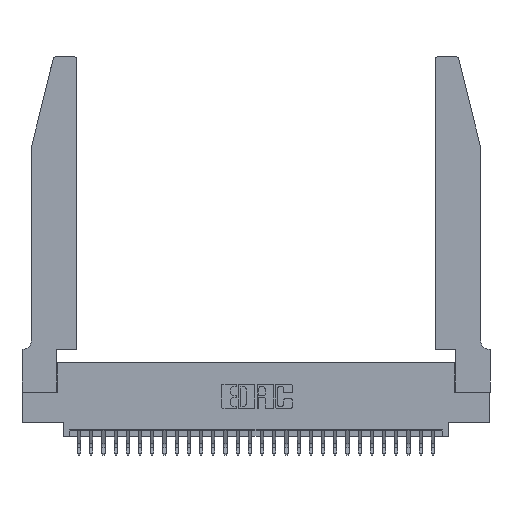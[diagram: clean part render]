
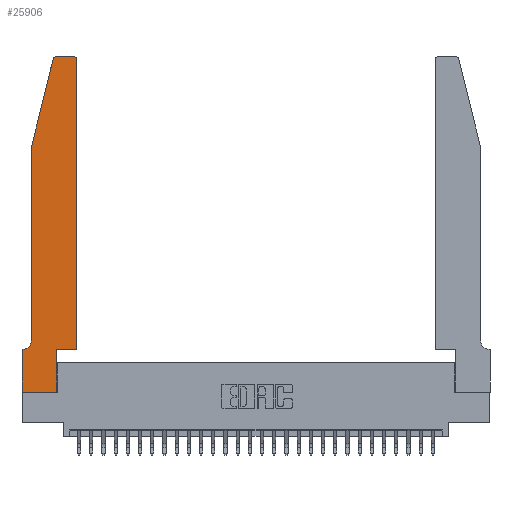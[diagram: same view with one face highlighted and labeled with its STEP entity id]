
A CAD part, top view. The second image highlights one B-rep face of the part: STEP entity #25906.
In plain terms, the highlighted planar face has unit normal (0, 0, 1).
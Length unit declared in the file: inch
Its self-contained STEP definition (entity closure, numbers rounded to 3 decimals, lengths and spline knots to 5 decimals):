
#276 = VECTOR ( 'NONE', #436, 39.37008 ) ;
#436 = DIRECTION ( 'NONE',  ( -1., 0., 0. ) ) ;
#448 = DIRECTION ( 'NONE',  ( 0., 0., 1. ) ) ;
#488 = EDGE_CURVE ( 'NONE', #23680, #1895, #4856, .T. ) ;
#511 = DIRECTION ( 'NONE',  ( 0., 0., 1. ) ) ;
#512 = DIRECTION ( 'NONE',  ( 1., 0., 0. ) ) ;
#603 = EDGE_CURVE ( 'NONE', #10189, #12084, #26690, .T. ) ;
#1034 = PLANE ( 'NONE',  #3310 ) ;
#1354 = DIRECTION ( 'NONE',  ( 0., 0., -1. ) ) ;
#1372 = CARTESIAN_POINT ( 'NONE',  ( 0.4505, 2.72, 0.37 ) ) ;
#1653 = LINE ( 'NONE', #19392, #18982 ) ;
#1687 = CARTESIAN_POINT ( 'NONE',  ( 0.284, 2.72, 0.37 ) ) ;
#1745 = EDGE_CURVE ( 'NONE', #4046, #21541, #2891, .T. ) ;
#1805 = VECTOR ( 'NONE', #23815, 39.37008 ) ;
#1895 = VERTEX_POINT ( 'NONE', #25128 ) ;
#2157 = VECTOR ( 'NONE', #3407, 39.37008 ) ;
#2166 = ORIENTED_EDGE ( 'NONE', *, *, #25799, .T. ) ;
#2244 = ORIENTED_EDGE ( 'NONE', *, *, #603, .T. ) ;
#2560 = EDGE_CURVE ( 'NONE', #2932, #22158, #19732, .T. ) ;
#2891 = LINE ( 'NONE', #7577, #8505 ) ;
#2932 = VERTEX_POINT ( 'NONE', #23604 ) ;
#3072 = EDGE_CURVE ( 'NONE', #22158, #4046, #1653, .T. ) ;
#3310 = AXIS2_PLACEMENT_3D ( 'NONE', #28834, #17592, #3482 ) ;
#3407 = DIRECTION ( 'NONE',  ( -1., 0., 0. ) ) ;
#3482 = DIRECTION ( 'NONE',  ( 1., 0., 0. ) ) ;
#3757 = CARTESIAN_POINT ( 'NONE',  ( 0.4205, 2.75, 0.37 ) ) ;
#4046 = VERTEX_POINT ( 'NONE', #18332 ) ;
#4339 = ORIENTED_EDGE ( 'NONE', *, *, #15029, .T. ) ;
#4535 = VERTEX_POINT ( 'NONE', #1372 ) ;
#4721 = CARTESIAN_POINT ( 'NONE',  ( 0., 0., 0.37 ) ) ;
#4856 = LINE ( 'NONE', #27720, #28850 ) ;
#5128 = ORIENTED_EDGE ( 'NONE', *, *, #22657, .T. ) ;
#5544 = CARTESIAN_POINT ( 'NONE',  ( 0.2865, 0.35, 0.37 ) ) ;
#5922 = CARTESIAN_POINT ( 'NONE',  ( 0.2605, 2.75, 0.37 ) ) ;
#6476 = CARTESIAN_POINT ( 'NONE',  ( 0.4505, 0.35, 0.37 ) ) ;
#7117 = AXIS2_PLACEMENT_3D ( 'NONE', #14786, #511, #17093 ) ;
#7577 = CARTESIAN_POINT ( 'NONE',  ( 0.0755, 2., 0.37 ) ) ;
#8505 = VECTOR ( 'NONE', #15034, 39.37008 ) ;
#8634 = VERTEX_POINT ( 'NONE', #3757 ) ;
#9232 = VECTOR ( 'NONE', #27565, 39.37008 ) ;
#9397 = CARTESIAN_POINT ( 'NONE',  ( 0.4505, 0.35, 0.37 ) ) ;
#10058 = LINE ( 'NONE', #5922, #2157 ) ;
#10189 = VERTEX_POINT ( 'NONE', #13034 ) ;
#10328 = CIRCLE ( 'NONE', #13252, 0.07 ) ;
#11136 = ORIENTED_EDGE ( 'NONE', *, *, #2560, .T. ) ;
#12084 = VERTEX_POINT ( 'NONE', #6476 ) ;
#12278 = VECTOR ( 'NONE', #24158, 39.37008 ) ;
#13034 = CARTESIAN_POINT ( 'NONE',  ( 0.2865, 0.35, 0.37 ) ) ;
#13252 = AXIS2_PLACEMENT_3D ( 'NONE', #15545, #1354, #17889 ) ;
#13412 = ORIENTED_EDGE ( 'NONE', *, *, #3072, .T. ) ;
#13718 = LINE ( 'NONE', #23833, #276 ) ;
#13802 = CARTESIAN_POINT ( 'NONE',  ( 0.4505, 0.35, 0.37 ) ) ;
#14420 = EDGE_CURVE ( 'NONE', #1895, #10189, #29874, .T. ) ;
#14786 = CARTESIAN_POINT ( 'NONE',  ( 0.4205, 2.72, 0.37 ) ) ;
#15029 = EDGE_CURVE ( 'NONE', #12084, #4535, #27680, .T. ) ;
#15034 = DIRECTION ( 'NONE',  ( 0., -1., 0. ) ) ;
#15545 = CARTESIAN_POINT ( 'NONE',  ( 0.0055, 0.42, 0.37 ) ) ;
#16138 = ORIENTED_EDGE ( 'NONE', *, *, #24060, .T. ) ;
#16481 = EDGE_CURVE ( 'NONE', #21570, #23680, #18293, .T. ) ;
#16972 = VERTEX_POINT ( 'NONE', #23539 ) ;
#17092 = DIRECTION ( 'NONE',  ( -0.239, -0.971, 0. ) ) ;
#17093 = DIRECTION ( 'NONE',  ( 1., 0., 0. ) ) ;
#17592 = DIRECTION ( 'NONE',  ( 0., 0., 1. ) ) ;
#17889 = DIRECTION ( 'NONE',  ( -1., 0., 0. ) ) ;
#18293 = LINE ( 'NONE', #4721, #19008 ) ;
#18332 = CARTESIAN_POINT ( 'NONE',  ( 0.0755, 2., 0.37 ) ) ;
#18870 = ORIENTED_EDGE ( 'NONE', *, *, #22479, .T. ) ;
#18982 = VECTOR ( 'NONE', #17092, 39.37008 ) ;
#19008 = VECTOR ( 'NONE', #27893, 39.37008 ) ;
#19392 = CARTESIAN_POINT ( 'NONE',  ( 0.0755, 2., 0.37 ) ) ;
#19732 = CIRCLE ( 'NONE', #29746, 0.03 ) ;
#20115 = DIRECTION ( 'NONE',  ( 1., 0., 0. ) ) ;
#20415 = CIRCLE ( 'NONE', #7117, 0.03 ) ;
#20974 = CARTESIAN_POINT ( 'NONE',  ( 0., 0., 0.37 ) ) ;
#21309 = ORIENTED_EDGE ( 'NONE', *, *, #14420, .T. ) ;
#21541 = VERTEX_POINT ( 'NONE', #22276 ) ;
#21570 = VERTEX_POINT ( 'NONE', #26904 ) ;
#21665 = ORIENTED_EDGE ( 'NONE', *, *, #488, .T. ) ;
#22158 = VERTEX_POINT ( 'NONE', #27063 ) ;
#22276 = CARTESIAN_POINT ( 'NONE',  ( 0.0755, 0.42, 0.37 ) ) ;
#22479 = EDGE_CURVE ( 'NONE', #16972, #21570, #13718, .T. ) ;
#22657 = EDGE_CURVE ( 'NONE', #8634, #2932, #10058, .T. ) ;
#23487 = ORIENTED_EDGE ( 'NONE', *, *, #1745, .T. ) ;
#23539 = CARTESIAN_POINT ( 'NONE',  ( 0.0055, 0.35, 0.37 ) ) ;
#23604 = CARTESIAN_POINT ( 'NONE',  ( 0.284, 2.75, 0.37 ) ) ;
#23680 = VERTEX_POINT ( 'NONE', #20974 ) ;
#23815 = DIRECTION ( 'NONE',  ( 1., 0., 0. ) ) ;
#23833 = CARTESIAN_POINT ( 'NONE',  ( 0.0755, 0.35, 0.37 ) ) ;
#24060 = EDGE_CURVE ( 'NONE', #21541, #16972, #10328, .T. ) ;
#24158 = DIRECTION ( 'NONE',  ( 0., 1., 0. ) ) ;
#25105 = FACE_OUTER_BOUND ( 'NONE', #29223, .T. ) ;
#25128 = CARTESIAN_POINT ( 'NONE',  ( 0.2865, 0., 0.37 ) ) ;
#25799 = EDGE_CURVE ( 'NONE', #4535, #8634, #20415, .T. ) ;
#25906 = ADVANCED_FACE ( 'NONE', ( #25105 ), #1034, .T. ) ;
#26690 = LINE ( 'NONE', #9397, #1805 ) ;
#26904 = CARTESIAN_POINT ( 'NONE',  ( 0., 0.35, 0.37 ) ) ;
#27063 = CARTESIAN_POINT ( 'NONE',  ( 0.25487, 2.72718, 0.37 ) ) ;
#27565 = DIRECTION ( 'NONE',  ( 0., 1., 0. ) ) ;
#27680 = LINE ( 'NONE', #13802, #9232 ) ;
#27720 = CARTESIAN_POINT ( 'NONE',  ( 0., 0., 0.37 ) ) ;
#27893 = DIRECTION ( 'NONE',  ( 0., -1., 0. ) ) ;
#28834 = CARTESIAN_POINT ( 'NONE',  ( 0., 0.35, 0.37 ) ) ;
#28850 = VECTOR ( 'NONE', #20115, 39.37008 ) ;
#29223 = EDGE_LOOP ( 'NONE', ( #5128, #11136, #13412, #23487, #16138, #18870, #30028, #21665, #21309, #2244, #4339, #2166 ) ) ;
#29746 = AXIS2_PLACEMENT_3D ( 'NONE', #1687, #448, #512 ) ;
#29874 = LINE ( 'NONE', #5544, #12278 ) ;
#30028 = ORIENTED_EDGE ( 'NONE', *, *, #16481, .T. ) ;
